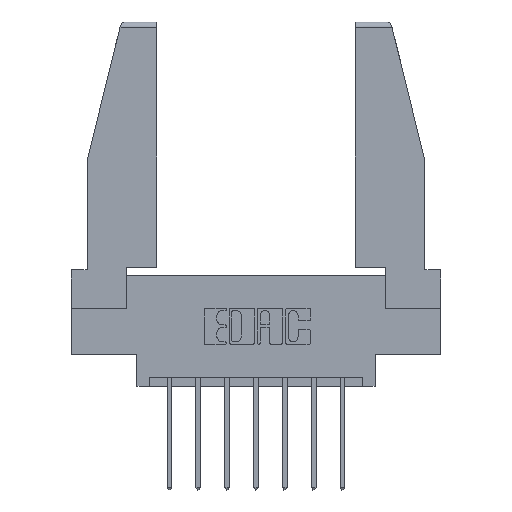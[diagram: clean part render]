
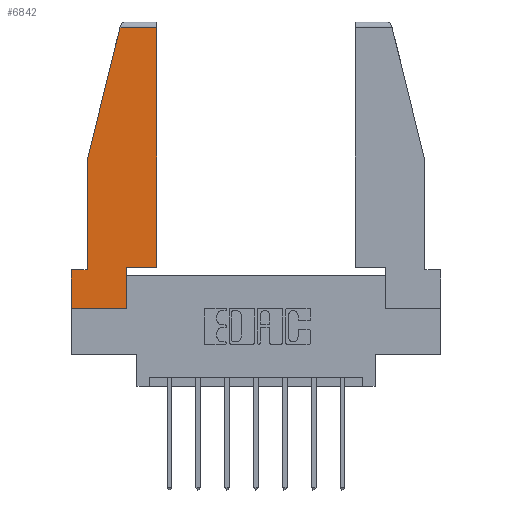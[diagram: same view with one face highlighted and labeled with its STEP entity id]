
A CAD part, top view. The second image highlights one B-rep face of the part: STEP entity #6842.
In plain terms, the highlighted planar face has unit normal (0, 0, 1).
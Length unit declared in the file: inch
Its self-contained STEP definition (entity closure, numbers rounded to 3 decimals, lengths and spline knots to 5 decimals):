
#15 = DIRECTION ( 'NONE',  ( 0., -1., 0. ) ) ;
#25 = LINE ( 'NONE', #9094, #7203 ) ;
#95 = AXIS2_PLACEMENT_3D ( 'NONE', #8316, #5477, #6421 ) ;
#159 = EDGE_CURVE ( 'NONE', #614, #2579, #8092, .T. ) ;
#160 = CARTESIAN_POINT ( 'NONE',  ( 0.2636, 1.52, 0. ) ) ;
#309 = EDGE_CURVE ( 'NONE', #1562, #5739, #25, .T. ) ;
#482 = CARTESIAN_POINT ( 'NONE',  ( 0.461, 0.223, 0. ) ) ;
#614 = VERTEX_POINT ( 'NONE', #7091 ) ;
#751 = LINE ( 'NONE', #5062, #6234 ) ;
#766 = VERTEX_POINT ( 'NONE', #160 ) ;
#1455 = DIRECTION ( 'NONE',  ( 0., 1., 0. ) ) ;
#1458 = DIRECTION ( 'NONE',  ( 1., 0., 0. ) ) ;
#1562 = VERTEX_POINT ( 'NONE', #7031 ) ;
#1947 = EDGE_CURVE ( 'NONE', #5739, #2690, #3949, .T. ) ;
#2190 = EDGE_CURVE ( 'NONE', #10468, #614, #751, .T. ) ;
#2217 = DIRECTION ( 'NONE',  ( 0., -1., 0. ) ) ;
#2290 = DIRECTION ( 'NONE',  ( 1., 0., 0. ) ) ;
#2432 = CARTESIAN_POINT ( 'NONE',  ( 0.461, 0.223, 0. ) ) ;
#2560 = LINE ( 'NONE', #10652, #5472 ) ;
#2579 = VERTEX_POINT ( 'NONE', #8253 ) ;
#2657 = ORIENTED_EDGE ( 'NONE', *, *, #2918, .T. ) ;
#2690 = VERTEX_POINT ( 'NONE', #2432 ) ;
#2918 = EDGE_CURVE ( 'NONE', #2579, #8997, #10768, .T. ) ;
#2962 = CARTESIAN_POINT ( 'NONE',  ( 0., 0., 0. ) ) ;
#3096 = CARTESIAN_POINT ( 'NONE',  ( 0.271, 1.55, 0. ) ) ;
#3527 = EDGE_CURVE ( 'NONE', #8997, #1562, #6655, .T. ) ;
#3949 = LINE ( 'NONE', #5375, #9880 ) ;
#3995 = CARTESIAN_POINT ( 'NONE',  ( 0.086, 0.8, 0. ) ) ;
#4043 = VECTOR ( 'NONE', #2290, 39.37008 ) ;
#4120 = EDGE_LOOP ( 'NONE', ( #4901, #8851, #12324, #9798, #7107, #2657, #4657, #10647, #12413 ) ) ;
#4565 = PLANE ( 'NONE',  #95 ) ;
#4590 = VECTOR ( 'NONE', #6953, 39.37008 ) ;
#4657 = ORIENTED_EDGE ( 'NONE', *, *, #3527, .T. ) ;
#4794 = DIRECTION ( 'NONE',  ( -1., 0., 0. ) ) ;
#4901 = ORIENTED_EDGE ( 'NONE', *, *, #11380, .T. ) ;
#5062 = CARTESIAN_POINT ( 'NONE',  ( 0.086, 0.8, 0. ) ) ;
#5375 = CARTESIAN_POINT ( 'NONE',  ( 0.297, 0.223, 0. ) ) ;
#5472 = VECTOR ( 'NONE', #4794, 39.37008 ) ;
#5477 = DIRECTION ( 'NONE',  ( 0., 0., 1. ) ) ;
#5739 = VERTEX_POINT ( 'NONE', #7959 ) ;
#5962 = EDGE_CURVE ( 'NONE', #766, #10468, #10069, .T. ) ;
#6234 = VECTOR ( 'NONE', #2217, 39.37008 ) ;
#6353 = VECTOR ( 'NONE', #15, 39.37008 ) ;
#6375 = VECTOR ( 'NONE', #1455, 39.37008 ) ;
#6421 = DIRECTION ( 'NONE',  ( 1., 0., 0. ) ) ;
#6655 = LINE ( 'NONE', #8114, #4043 ) ;
#6842 = ADVANCED_FACE ( 'NONE', ( #7611 ), #4565, .T. ) ;
#6953 = DIRECTION ( 'NONE',  ( -0.239, -0.971, 0. ) ) ;
#7031 = CARTESIAN_POINT ( 'NONE',  ( 0.297, 0., 0. ) ) ;
#7091 = CARTESIAN_POINT ( 'NONE',  ( 0.086, 0.21, 0. ) ) ;
#7107 = ORIENTED_EDGE ( 'NONE', *, *, #159, .T. ) ;
#7203 = VECTOR ( 'NONE', #7604, 39.37008 ) ;
#7284 = LINE ( 'NONE', #482, #6375 ) ;
#7539 = EDGE_CURVE ( 'NONE', #9452, #766, #2560, .T. ) ;
#7604 = DIRECTION ( 'NONE',  ( 0., 1., 0. ) ) ;
#7611 = FACE_OUTER_BOUND ( 'NONE', #4120, .T. ) ;
#7959 = CARTESIAN_POINT ( 'NONE',  ( 0.297, 0.223, 0. ) ) ;
#8092 = LINE ( 'NONE', #12448, #11298 ) ;
#8114 = CARTESIAN_POINT ( 'NONE',  ( 0., 0., 0. ) ) ;
#8253 = CARTESIAN_POINT ( 'NONE',  ( 0., 0.21, 0. ) ) ;
#8316 = CARTESIAN_POINT ( 'NONE',  ( 0., 0., 0. ) ) ;
#8851 = ORIENTED_EDGE ( 'NONE', *, *, #7539, .T. ) ;
#8997 = VERTEX_POINT ( 'NONE', #2962 ) ;
#9094 = CARTESIAN_POINT ( 'NONE',  ( 0.297, 0., 0. ) ) ;
#9310 = CARTESIAN_POINT ( 'NONE',  ( 0.461, 1.52, 0. ) ) ;
#9452 = VERTEX_POINT ( 'NONE', #9310 ) ;
#9798 = ORIENTED_EDGE ( 'NONE', *, *, #2190, .T. ) ;
#9880 = VECTOR ( 'NONE', #1458, 39.37008 ) ;
#10069 = LINE ( 'NONE', #3096, #4590 ) ;
#10468 = VERTEX_POINT ( 'NONE', #3995 ) ;
#10615 = DIRECTION ( 'NONE',  ( -1., 0., 0. ) ) ;
#10622 = CARTESIAN_POINT ( 'NONE',  ( 0., 0.21, 0. ) ) ;
#10647 = ORIENTED_EDGE ( 'NONE', *, *, #309, .T. ) ;
#10652 = CARTESIAN_POINT ( 'NONE',  ( 0., 1.52, 0. ) ) ;
#10768 = LINE ( 'NONE', #10622, #6353 ) ;
#11298 = VECTOR ( 'NONE', #10615, 39.37008 ) ;
#11380 = EDGE_CURVE ( 'NONE', #2690, #9452, #7284, .T. ) ;
#12324 = ORIENTED_EDGE ( 'NONE', *, *, #5962, .T. ) ;
#12413 = ORIENTED_EDGE ( 'NONE', *, *, #1947, .T. ) ;
#12448 = CARTESIAN_POINT ( 'NONE',  ( 0., 0.21, 0. ) ) ;
